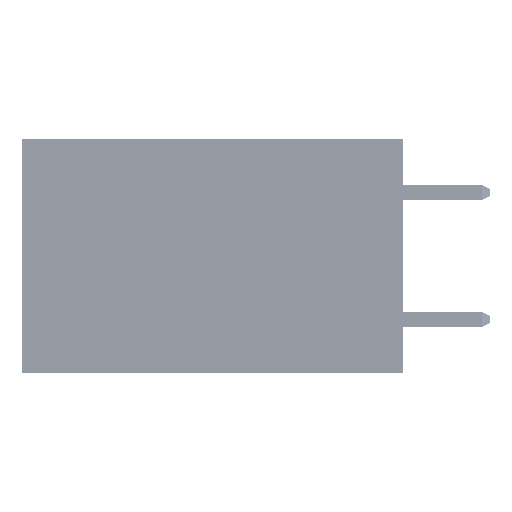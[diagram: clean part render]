
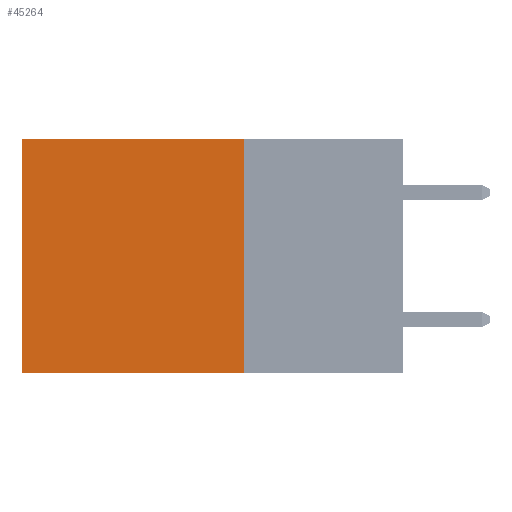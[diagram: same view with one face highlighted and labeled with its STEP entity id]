
A CAD part, left-side view. The second image highlights one B-rep face of the part: STEP entity #45264.
In plain terms, the highlighted planar face has unit normal (-1, 0, 0).
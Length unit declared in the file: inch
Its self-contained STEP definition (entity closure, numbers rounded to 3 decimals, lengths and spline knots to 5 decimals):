
#1154 = DIRECTION ( 'NONE',  ( 0., 0., -1. ) ) ;
#3726 = VECTOR ( 'NONE', #43107, 39.37008 ) ;
#3871 = ORIENTED_EDGE ( 'NONE', *, *, #15519, .F. ) ;
#4681 = ORIENTED_EDGE ( 'NONE', *, *, #5081, .T. ) ;
#4824 = VECTOR ( 'NONE', #20134, 39.37008 ) ;
#5003 = LINE ( 'NONE', #39849, #26353 ) ;
#5081 = EDGE_CURVE ( 'NONE', #23415, #23905, #45073, .T. ) ;
#5988 = CARTESIAN_POINT ( 'NONE',  ( 0.2875, 0.25, -0.37 ) ) ;
#7156 = AXIS2_PLACEMENT_3D ( 'NONE', #18945, #46904, #22942 ) ;
#7504 = VERTEX_POINT ( 'NONE', #5988 ) ;
#9329 = EDGE_LOOP ( 'NONE', ( #4681, #11067, #3871, #28922 ) ) ;
#11067 = ORIENTED_EDGE ( 'NONE', *, *, #29114, .F. ) ;
#11917 = DIRECTION ( 'NONE',  ( 0., 1., 0. ) ) ;
#12122 = CARTESIAN_POINT ( 'NONE',  ( 0.2875, 0.25, 0. ) ) ;
#12950 = EDGE_CURVE ( 'NONE', #51047, #23415, #47437, .T. ) ;
#15189 = CARTESIAN_POINT ( 'NONE',  ( 0.2875, 0.6, 0. ) ) ;
#15519 = EDGE_CURVE ( 'NONE', #51047, #7504, #50974, .T. ) ;
#18945 = CARTESIAN_POINT ( 'NONE',  ( 0.2875, 0.25, 0. ) ) ;
#20134 = DIRECTION ( 'NONE',  ( 0., 1., 0. ) ) ;
#22942 = DIRECTION ( 'NONE',  ( 0., 0., -1. ) ) ;
#23415 = VERTEX_POINT ( 'NONE', #25641 ) ;
#23905 = VERTEX_POINT ( 'NONE', #44450 ) ;
#25641 = CARTESIAN_POINT ( 'NONE',  ( 0.2875, 0.6, 0. ) ) ;
#26353 = VECTOR ( 'NONE', #11917, 39.37008 ) ;
#28922 = ORIENTED_EDGE ( 'NONE', *, *, #12950, .T. ) ;
#29114 = EDGE_CURVE ( 'NONE', #7504, #23905, #5003, .T. ) ;
#33700 = CARTESIAN_POINT ( 'NONE',  ( 0.2875, 0.25, 0. ) ) ;
#37246 = CARTESIAN_POINT ( 'NONE',  ( 0.2875, 0.25, 0. ) ) ;
#38848 = PLANE ( 'NONE',  #7156 ) ;
#39849 = CARTESIAN_POINT ( 'NONE',  ( 0.2875, 0.25, -0.37 ) ) ;
#42878 = VECTOR ( 'NONE', #1154, 39.37008 ) ;
#43107 = DIRECTION ( 'NONE',  ( 0., 0., -1. ) ) ;
#44450 = CARTESIAN_POINT ( 'NONE',  ( 0.2875, 0.6, -0.37 ) ) ;
#45073 = LINE ( 'NONE', #15189, #3726 ) ;
#45264 = ADVANCED_FACE ( 'NONE', ( #46609 ), #38848, .F. ) ;
#46609 = FACE_OUTER_BOUND ( 'NONE', #9329, .T. ) ;
#46904 = DIRECTION ( 'NONE',  ( 1., 0., 0. ) ) ;
#47437 = LINE ( 'NONE', #12122, #4824 ) ;
#50974 = LINE ( 'NONE', #37246, #42878 ) ;
#51047 = VERTEX_POINT ( 'NONE', #33700 ) ;
